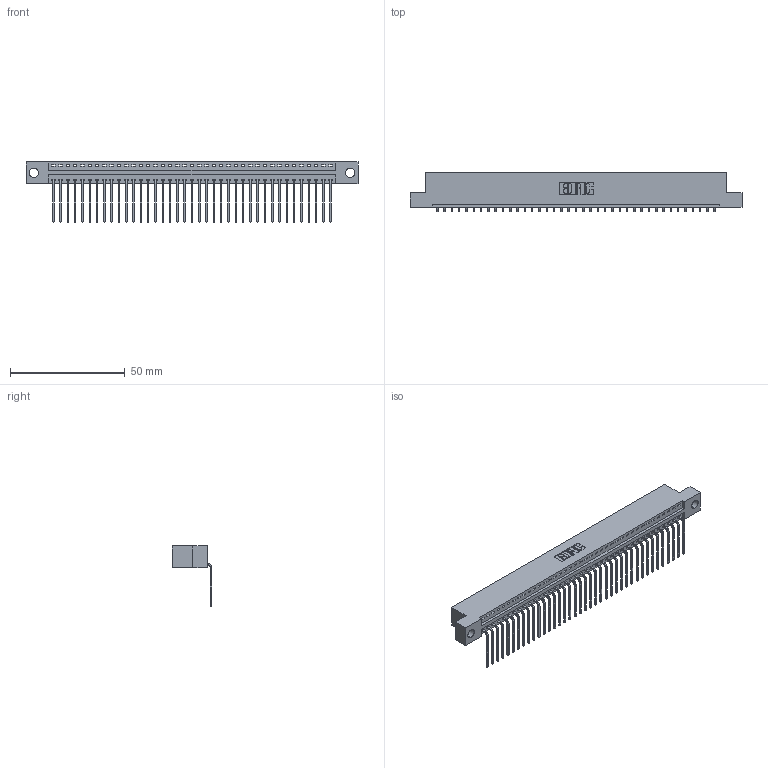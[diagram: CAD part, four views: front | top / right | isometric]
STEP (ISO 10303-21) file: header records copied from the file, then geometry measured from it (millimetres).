
FILE_DESCRIPTION (( 'STEP AP203' ), '1' );
FILE_NAME ('346-039-559-104.STEP', '2022-05-07T08:07:06', ( '' ), ( '' ), 'SwSTEP 2.0', 'SolidWorks 2020', '' );
FILE_SCHEMA (( 'CONFIG_CONTROL_DESIGN' ));
Length unit declared in the file: inch
Products named in the file (3): 345-292-001_558 559 Tail - 1; 346 Part_Flush Mounting Lugs - 0.156 Dia-TH; 346-039-559-104
Assembly tree (40 placements, depth 2):
  346-039-559-104
    346 Part_Flush Mounting Lugs - 0.156 Dia-TH
    345-292-001_558 559 Tail - 1  x39
Bounding box: 144.4 x 17.08 x 26.16 mm (x, y, z)
Volume: 13825.5 mm3; surface area: 17860.2 mm2
Topology: 40 solids, 40 shells, 2476 faces, 7463 edges, 4922 vertices
Faces by surface type: plane 1728, cylinder 748
Entity records: 25111 total; most frequent: CARTESIAN_POINT 4315, ORIENTED_EDGE 4286, DIRECTION 3809, EDGE_CURVE 2143, VECTOR 1855, LINE 1855, VERTEX_POINT 1426, AXIS2_PLACEMENT_3D 977
